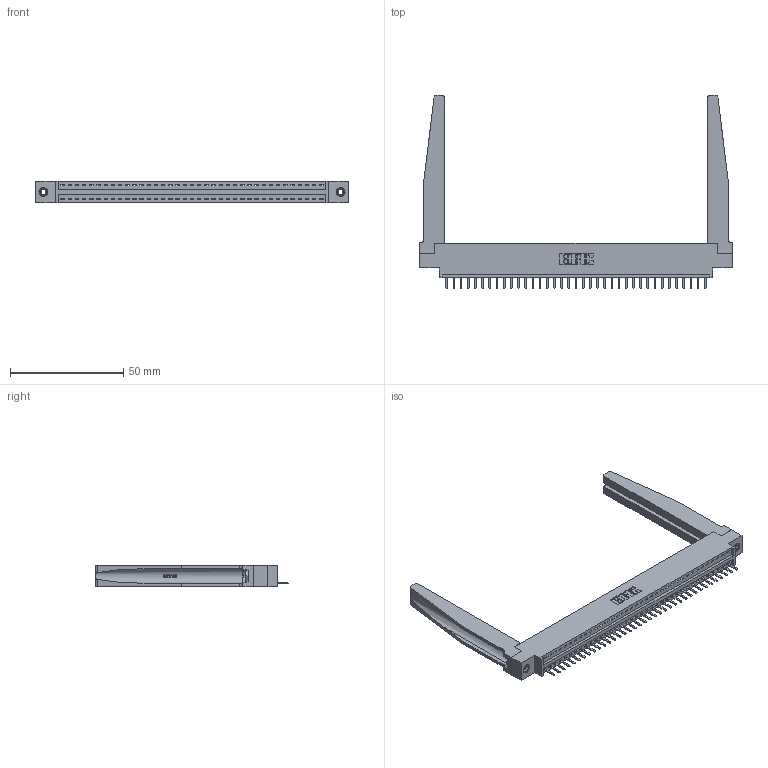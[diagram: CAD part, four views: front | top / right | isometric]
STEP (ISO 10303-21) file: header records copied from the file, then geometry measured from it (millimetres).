
FILE_DESCRIPTION (( 'STEP AP203' ), '1' );
FILE_NAME ('346-037-520-678.STEP', '2022-05-07T02:19:15', ( '' ), ( '' ), 'SwSTEP 2.0', 'SolidWorks 2020', '' );
FILE_SCHEMA (( 'CONFIG_CONTROL_DESIGN' ));
Length unit declared in the file: inch
Products named in the file (5): 345-292-001_345-293-120; 346 Part_0.170 Offset - 0.156 Dia-TH; 345-250-001_345-250-001-102; 346-037-520-678; 346-220-078_345-220-078
Assembly tree (42 placements, depth 2):
  346-037-520-678
    346 Part_0.170 Offset - 0.156 Dia-TH
    345-292-001_345-293-120  x37
    346-220-078_345-220-078  x2
    345-250-001_345-250-001-102  x2
Bounding box: 138.05 x 85.29 x 9.4 mm (x, y, z)
Volume: 19809.6 mm3; surface area: 22447.8 mm2
Topology: 42 solids, 42 shells, 2668 faces, 7793 edges, 5086 vertices
Faces by surface type: plane 1790, cylinder 826, bspline 36, cone 12, torus 4
Entity records: 29046 total; most frequent: CARTESIAN_POINT 5908, ORIENTED_EDGE 4754, DIRECTION 4189, EDGE_CURVE 2377, VECTOR 1999, LINE 1999, VERTEX_POINT 1576, AXIS2_PLACEMENT_3D 1095
